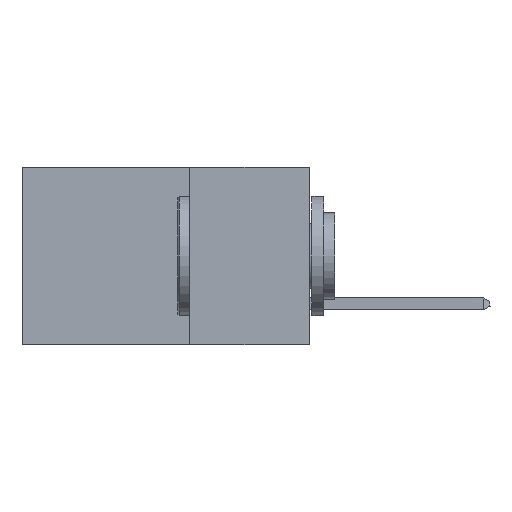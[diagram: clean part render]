
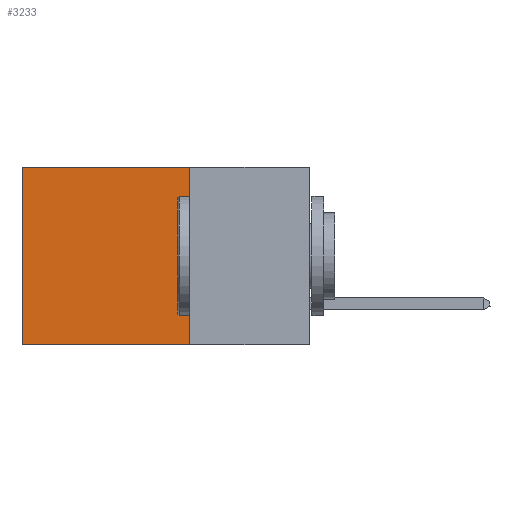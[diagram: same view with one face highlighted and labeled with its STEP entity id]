
A CAD part, left-side view. The second image highlights one B-rep face of the part: STEP entity #3233.
In plain terms, the highlighted planar face has unit normal (-1, 0, 0).
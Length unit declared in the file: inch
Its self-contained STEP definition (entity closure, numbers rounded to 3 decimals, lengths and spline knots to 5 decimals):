
#14 = ORIENTED_EDGE ( 'NONE', *, *, #2766, .T. ) ;
#580 = VERTEX_POINT ( 'NONE', #4863 ) ;
#760 = DIRECTION ( 'NONE',  ( 0., 1., 0. ) ) ;
#919 = LINE ( 'NONE', #8151, #14045 ) ;
#1153 = VECTOR ( 'NONE', #760, 39.37008 ) ;
#2059 = DIRECTION ( 'NONE',  ( 0., 0., -1. ) ) ;
#2764 = VERTEX_POINT ( 'NONE', #18637 ) ;
#2766 = EDGE_CURVE ( 'NONE', #10752, #2764, #919, .T. ) ;
#3233 = ADVANCED_FACE ( 'NONE', ( #3351 ), #20374, .F. ) ;
#3319 = ORIENTED_EDGE ( 'NONE', *, *, #16872, .F. ) ;
#3351 = FACE_OUTER_BOUND ( 'NONE', #15852, .T. ) ;
#4863 = CARTESIAN_POINT ( 'NONE',  ( 0.2875, 0.25, -0.37 ) ) ;
#5123 = DIRECTION ( 'NONE',  ( 0., 1., 0. ) ) ;
#6338 = CARTESIAN_POINT ( 'NONE',  ( 0.2875, 0.25, 0. ) ) ;
#6601 = LINE ( 'NONE', #8544, #19500 ) ;
#8051 = VECTOR ( 'NONE', #5123, 39.37008 ) ;
#8151 = CARTESIAN_POINT ( 'NONE',  ( 0.2875, 0.6, 0. ) ) ;
#8221 = CARTESIAN_POINT ( 'NONE',  ( 0.2875, 0.25, -0.37 ) ) ;
#8544 = CARTESIAN_POINT ( 'NONE',  ( 0.2875, 0.25, 0. ) ) ;
#9460 = DIRECTION ( 'NONE',  ( 0., 0., -1. ) ) ;
#9937 = VERTEX_POINT ( 'NONE', #16043 ) ;
#10752 = VERTEX_POINT ( 'NONE', #15896 ) ;
#12554 = DIRECTION ( 'NONE',  ( 1., 0., 0. ) ) ;
#13176 = AXIS2_PLACEMENT_3D ( 'NONE', #6338, #12554, #9460 ) ;
#13266 = LINE ( 'NONE', #14674, #8051 ) ;
#14045 = VECTOR ( 'NONE', #17646, 39.37008 ) ;
#14674 = CARTESIAN_POINT ( 'NONE',  ( 0.2875, 0.25, 0. ) ) ;
#15034 = EDGE_CURVE ( 'NONE', #9937, #580, #6601, .T. ) ;
#15467 = LINE ( 'NONE', #8221, #1153 ) ;
#15852 = EDGE_LOOP ( 'NONE', ( #14, #3319, #17461, #19824 ) ) ;
#15896 = CARTESIAN_POINT ( 'NONE',  ( 0.2875, 0.6, 0. ) ) ;
#16043 = CARTESIAN_POINT ( 'NONE',  ( 0.2875, 0.25, 0. ) ) ;
#16827 = EDGE_CURVE ( 'NONE', #9937, #10752, #13266, .T. ) ;
#16872 = EDGE_CURVE ( 'NONE', #580, #2764, #15467, .T. ) ;
#17461 = ORIENTED_EDGE ( 'NONE', *, *, #15034, .F. ) ;
#17646 = DIRECTION ( 'NONE',  ( 0., 0., -1. ) ) ;
#18637 = CARTESIAN_POINT ( 'NONE',  ( 0.2875, 0.6, -0.37 ) ) ;
#19500 = VECTOR ( 'NONE', #2059, 39.37008 ) ;
#19824 = ORIENTED_EDGE ( 'NONE', *, *, #16827, .T. ) ;
#20374 = PLANE ( 'NONE',  #13176 ) ;
